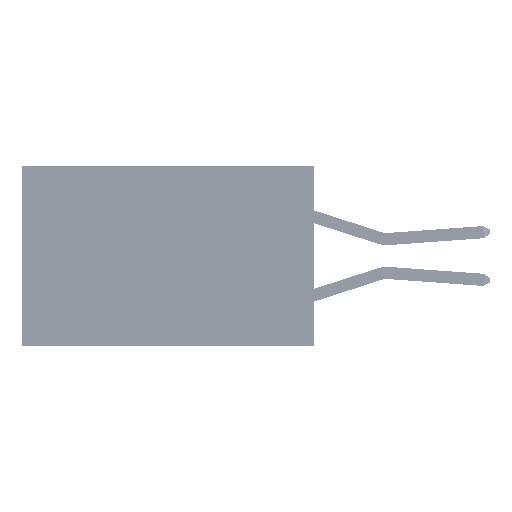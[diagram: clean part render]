
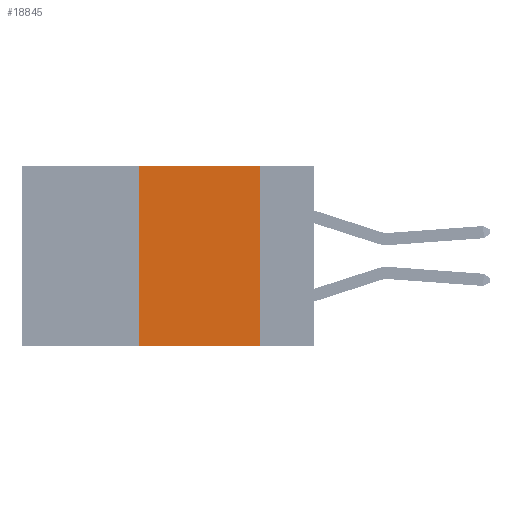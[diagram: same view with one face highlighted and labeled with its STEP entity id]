
A CAD part, left-side view. The second image highlights one B-rep face of the part: STEP entity #18845.
In plain terms, the highlighted planar face has unit normal (-1, 0, 0).
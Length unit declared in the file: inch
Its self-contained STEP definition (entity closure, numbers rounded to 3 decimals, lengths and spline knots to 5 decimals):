
#5060 = AXIS2_PLACEMENT_3D ( 'NONE', #8922, #36539, #16250 ) ;
#5334 = LINE ( 'NONE', #33346, #29050 ) ;
#6850 = VERTEX_POINT ( 'NONE', #17745 ) ;
#7594 = CARTESIAN_POINT ( 'NONE',  ( 0., 0.6, 0. ) ) ;
#8039 = VERTEX_POINT ( 'NONE', #41250 ) ;
#8262 = DIRECTION ( 'NONE',  ( 0., -1., 0. ) ) ;
#8922 = CARTESIAN_POINT ( 'NONE',  ( 0., 0.6, 0. ) ) ;
#12765 = PLANE ( 'NONE',  #5060 ) ;
#13170 = CARTESIAN_POINT ( 'NONE',  ( 0., 0.11, -0.37 ) ) ;
#14248 = LINE ( 'NONE', #19775, #16079 ) ;
#16079 = VECTOR ( 'NONE', #31284, 39.37008 ) ;
#16250 = DIRECTION ( 'NONE',  ( 0., 0., -1. ) ) ;
#17745 = CARTESIAN_POINT ( 'NONE',  ( 0., 0.36, -0.37 ) ) ;
#18845 = ADVANCED_FACE ( 'NONE', ( #19845 ), #12765, .F. ) ;
#19507 = ORIENTED_EDGE ( 'NONE', *, *, #48683, .F. ) ;
#19775 = CARTESIAN_POINT ( 'NONE',  ( 0., 0.6, -0.37 ) ) ;
#19845 = FACE_OUTER_BOUND ( 'NONE', #24398, .T. ) ;
#21003 = ORIENTED_EDGE ( 'NONE', *, *, #23209, .F. ) ;
#23209 = EDGE_CURVE ( 'NONE', #6850, #8039, #42381, .T. ) ;
#24398 = EDGE_LOOP ( 'NONE', ( #19507, #32282, #21003, #40608 ) ) ;
#25381 = DIRECTION ( 'NONE',  ( 0., 0., -1. ) ) ;
#26326 = VECTOR ( 'NONE', #30405, 39.37008 ) ;
#29050 = VECTOR ( 'NONE', #25381, 39.37008 ) ;
#30022 = LINE ( 'NONE', #7594, #49781 ) ;
#30069 = CARTESIAN_POINT ( 'NONE',  ( 0., 0.36, 0. ) ) ;
#30405 = DIRECTION ( 'NONE',  ( 0., 0., 1. ) ) ;
#31284 = DIRECTION ( 'NONE',  ( 0., -1., 0. ) ) ;
#32282 = ORIENTED_EDGE ( 'NONE', *, *, #39855, .F. ) ;
#33346 = CARTESIAN_POINT ( 'NONE',  ( 0., 0.11, 0. ) ) ;
#34240 = CARTESIAN_POINT ( 'NONE',  ( 0., 0.11, 0. ) ) ;
#35110 = VERTEX_POINT ( 'NONE', #34240 ) ;
#35604 = EDGE_CURVE ( 'NONE', #6850, #42591, #14248, .T. ) ;
#36539 = DIRECTION ( 'NONE',  ( 1., 0., 0. ) ) ;
#39855 = EDGE_CURVE ( 'NONE', #8039, #35110, #30022, .T. ) ;
#40608 = ORIENTED_EDGE ( 'NONE', *, *, #35604, .T. ) ;
#41250 = CARTESIAN_POINT ( 'NONE',  ( 0., 0.36, 0. ) ) ;
#42381 = LINE ( 'NONE', #30069, #26326 ) ;
#42591 = VERTEX_POINT ( 'NONE', #13170 ) ;
#48683 = EDGE_CURVE ( 'NONE', #35110, #42591, #5334, .T. ) ;
#49781 = VECTOR ( 'NONE', #8262, 39.37008 ) ;
